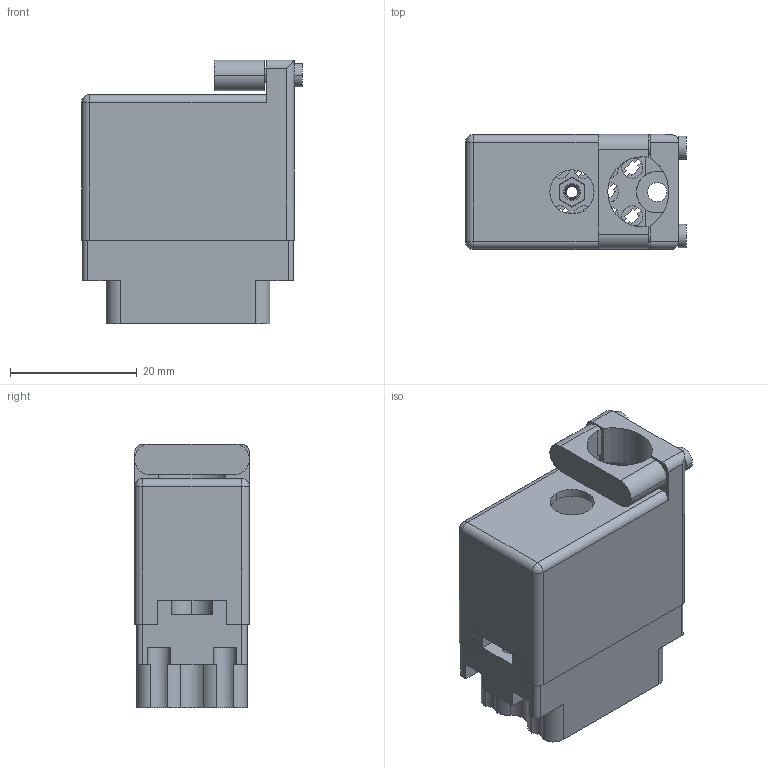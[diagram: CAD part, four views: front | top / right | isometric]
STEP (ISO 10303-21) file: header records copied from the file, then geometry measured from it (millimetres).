
FILE_DESCRIPTION (( 'STEP AP203' ), '1' );
FILE_NAME ('519-014-000-366.STEP', '2020-03-02T19:55:35', ( '' ), ( '' ), 'SwSTEP 2.0', 'SolidWorks 2016', '' );
FILE_SCHEMA (( 'CONFIG_CONTROL_DESIGN' ));
Length unit declared in the file: inch
Products named in the file (4): 516-230-001_Metal - 020 Top Entry; 516-252-025-100_516-252-025-100; 519-014-000-366; 519 Plug Insulator_014
Assembly tree (3 placements, depth 2):
  519-014-000-366
    519 Plug Insulator_014
    516-252-025-100_516-252-025-100
    516-230-001_Metal - 020 Top Entry
Bounding box: 34.92 x 18.16 x 41.71 mm (x, y, z)
Volume: 8859.9 mm3; surface area: 12364.7 mm2
Topology: 3 solids, 3 shells, 615 faces, 1774 edges, 1173 vertices
Faces by surface type: plane 371, cylinder 228, cone 11, bspline 3, sphere 2
Entity records: 23294 total; most frequent: CARTESIAN_POINT 6320, ORIENTED_EDGE 3544, DIRECTION 3433, EDGE_CURVE 1772, VECTOR 1223, LINE 1223, VERTEX_POINT 1173, AXIS2_PLACEMENT_3D 1105
